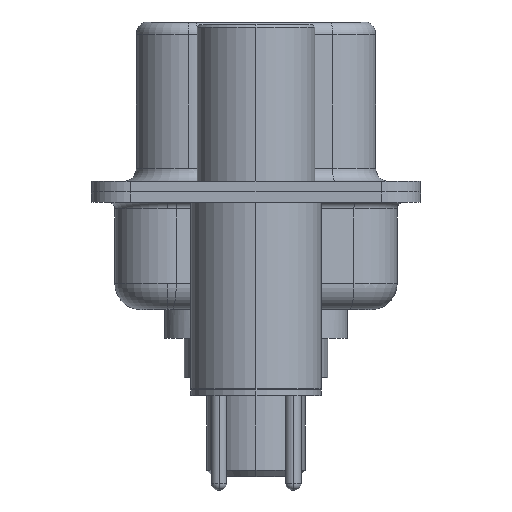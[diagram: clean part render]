
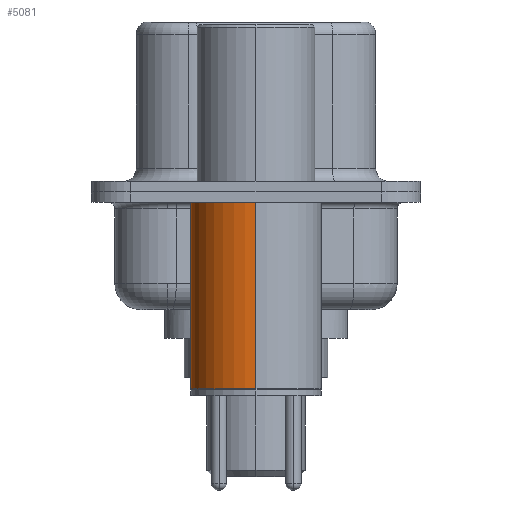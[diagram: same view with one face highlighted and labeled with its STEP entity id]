
A CAD part, left-side view. The second image highlights one B-rep face of the part: STEP entity #5081.
In plain terms, the highlighted cylindrical face has radius 2.5 mm (diameter 5 mm), a partial arc.
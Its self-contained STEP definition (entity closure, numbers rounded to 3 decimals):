
#1087 = EDGE_CURVE ( 'NONE', #14521, #20965, #11410, .T. ) ;
#1655 = DIRECTION ( 'NONE',  ( 0., 0., 1. ) ) ;
#2342 = ORIENTED_EDGE ( 'NONE', *, *, #17877, .F. ) ;
#3990 = EDGE_CURVE ( 'NONE', #16121, #14521, #11821, .T. ) ;
#5081 = ADVANCED_FACE ( 'NONE', ( #16758 ), #11272, .T. ) ;
#5663 = DIRECTION ( 'NONE',  ( 0., 0., 1. ) ) ;
#5762 = ORIENTED_EDGE ( 'NONE', *, *, #1087, .T. ) ;
#5940 = CARTESIAN_POINT ( 'NONE',  ( 2.5, 0., -7.525 ) ) ;
#6504 = VECTOR ( 'NONE', #1655, 1000. ) ;
#8557 = CARTESIAN_POINT ( 'NONE',  ( 0., 0., 0.581 ) ) ;
#9736 = CARTESIAN_POINT ( 'NONE',  ( 2.5, 0., 0.581 ) ) ;
#9976 = DIRECTION ( 'NONE',  ( 1., 0., 0. ) ) ;
#10048 = DIRECTION ( 'NONE',  ( 0., 0., 1. ) ) ;
#10890 = VERTEX_POINT ( 'NONE', #17324 ) ;
#10985 = AXIS2_PLACEMENT_3D ( 'NONE', #8557, #10048, #9976 ) ;
#11249 = DIRECTION ( 'NONE',  ( 1., 0., 0. ) ) ;
#11272 = CYLINDRICAL_SURFACE ( 'NONE', #10985, 2.5 ) ;
#11410 = LINE ( 'NONE', #19009, #20211 ) ;
#11776 = DIRECTION ( 'NONE',  ( 0., 0., 1. ) ) ;
#11821 = CIRCLE ( 'NONE', #16426, 2.5 ) ;
#12212 = CARTESIAN_POINT ( 'NONE',  ( 0., 0., -7.525 ) ) ;
#12262 = DIRECTION ( 'NONE',  ( 0., 0., 1. ) ) ;
#13898 = EDGE_LOOP ( 'NONE', ( #16560, #5762, #2342, #14554 ) ) ;
#14521 = VERTEX_POINT ( 'NONE', #21002 ) ;
#14554 = ORIENTED_EDGE ( 'NONE', *, *, #14600, .F. ) ;
#14600 = EDGE_CURVE ( 'NONE', #16121, #10890, #20079, .T. ) ;
#15447 = CARTESIAN_POINT ( 'NONE',  ( 0., 0., -0.4 ) ) ;
#16121 = VERTEX_POINT ( 'NONE', #5940 ) ;
#16235 = AXIS2_PLACEMENT_3D ( 'NONE', #15447, #5663, #17076 ) ;
#16426 = AXIS2_PLACEMENT_3D ( 'NONE', #12212, #12262, #11249 ) ;
#16560 = ORIENTED_EDGE ( 'NONE', *, *, #3990, .T. ) ;
#16758 = FACE_OUTER_BOUND ( 'NONE', #13898, .T. ) ;
#17009 = CARTESIAN_POINT ( 'NONE',  ( -2.5, 0., -0.4 ) ) ;
#17076 = DIRECTION ( 'NONE',  ( 1., 0., 0. ) ) ;
#17324 = CARTESIAN_POINT ( 'NONE',  ( 2.5, 0., -0.4 ) ) ;
#17877 = EDGE_CURVE ( 'NONE', #10890, #20965, #19546, .T. ) ;
#19009 = CARTESIAN_POINT ( 'NONE',  ( -2.5, 0., 0.581 ) ) ;
#19546 = CIRCLE ( 'NONE', #16235, 2.5 ) ;
#20079 = LINE ( 'NONE', #9736, #6504 ) ;
#20211 = VECTOR ( 'NONE', #11776, 1000. ) ;
#20965 = VERTEX_POINT ( 'NONE', #17009 ) ;
#21002 = CARTESIAN_POINT ( 'NONE',  ( -2.5, 0., -7.525 ) ) ;
